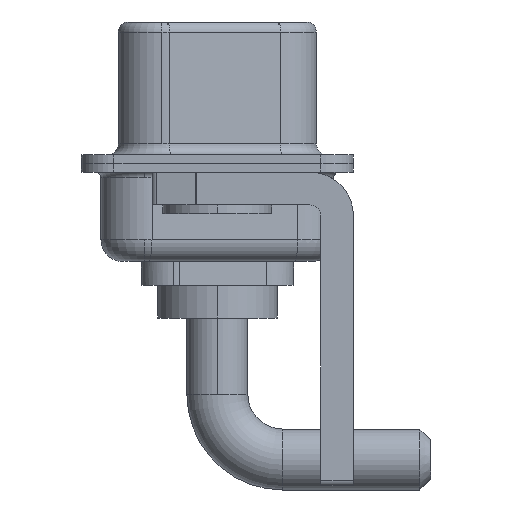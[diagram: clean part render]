
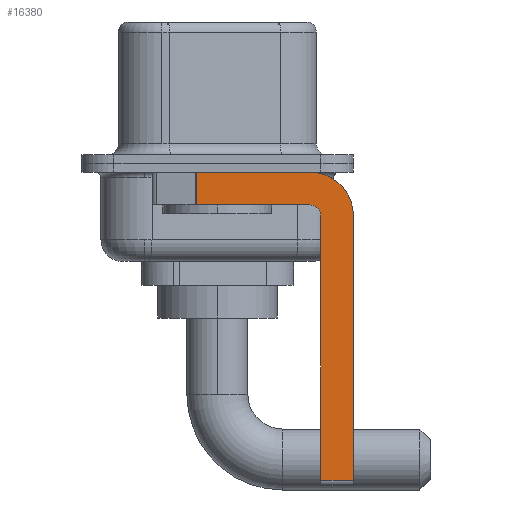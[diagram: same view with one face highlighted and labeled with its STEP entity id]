
A CAD part, left-side view. The second image highlights one B-rep face of the part: STEP entity #16380.
In plain terms, the highlighted planar face has unit normal (-1, 0, 0).
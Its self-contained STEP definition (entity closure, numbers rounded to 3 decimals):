
#33 = CARTESIAN_POINT ( 'NONE',  ( -2.9, -4.75, -14.55 ) ) ;
#86 = CIRCLE ( 'NONE', #16404, 2. ) ;
#243 = EDGE_CURVE ( 'NONE', #2593, #774, #3225, .T. ) ;
#257 = CARTESIAN_POINT ( 'NONE',  ( -2.9, -4.25, -1.9 ) ) ;
#627 = AXIS2_PLACEMENT_3D ( 'NONE', #12293, #13419, #5666 ) ;
#739 = VERTEX_POINT ( 'NONE', #6500 ) ;
#774 = VERTEX_POINT ( 'NONE', #1384 ) ;
#1222 = ORIENTED_EDGE ( 'NONE', *, *, #3602, .F. ) ;
#1384 = CARTESIAN_POINT ( 'NONE',  ( -2.9, 0.978, -1.9 ) ) ;
#1558 = ORIENTED_EDGE ( 'NONE', *, *, #5678, .F. ) ;
#1972 = VECTOR ( 'NONE', #9019, 1000. ) ;
#2199 = CARTESIAN_POINT ( 'NONE',  ( -2.9, -4.25, -2.4 ) ) ;
#2265 = VERTEX_POINT ( 'NONE', #33 ) ;
#2532 = DIRECTION ( 'NONE',  ( 0., 0., -1. ) ) ;
#2593 = VERTEX_POINT ( 'NONE', #11595 ) ;
#2694 = EDGE_CURVE ( 'NONE', #8889, #739, #14136, .T. ) ;
#3225 = LINE ( 'NONE', #7129, #10905 ) ;
#3522 = VERTEX_POINT ( 'NONE', #14858 ) ;
#3602 = EDGE_CURVE ( 'NONE', #3522, #14218, #7430, .T. ) ;
#3808 = PLANE ( 'NONE',  #4831 ) ;
#4029 = DIRECTION ( 'NONE',  ( 0., 0., -1. ) ) ;
#4514 = ORIENTED_EDGE ( 'NONE', *, *, #5252, .F. ) ;
#4831 = AXIS2_PLACEMENT_3D ( 'NONE', #2199, #8995, #2532 ) ;
#5252 = EDGE_CURVE ( 'NONE', #2593, #13153, #6380, .T. ) ;
#5563 = ORIENTED_EDGE ( 'NONE', *, *, #8252, .T. ) ;
#5666 = DIRECTION ( 'NONE',  ( 0., 0., 1. ) ) ;
#5678 = EDGE_CURVE ( 'NONE', #14218, #774, #8286, .T. ) ;
#5967 = VECTOR ( 'NONE', #7165, 1000. ) ;
#6380 = LINE ( 'NONE', #10470, #9667 ) ;
#6500 = CARTESIAN_POINT ( 'NONE',  ( -2.9, -6.25, -14.55 ) ) ;
#7129 = CARTESIAN_POINT ( 'NONE',  ( -2.9, 0.978, -1.9 ) ) ;
#7165 = DIRECTION ( 'NONE',  ( 0., 1., 0. ) ) ;
#7430 = CIRCLE ( 'NONE', #627, 0.5 ) ;
#7485 = DIRECTION ( 'NONE',  ( 0., -1., 0. ) ) ;
#8115 = ORIENTED_EDGE ( 'NONE', *, *, #243, .T. ) ;
#8252 = EDGE_CURVE ( 'NONE', #2265, #739, #16117, .T. ) ;
#8286 = LINE ( 'NONE', #16116, #5967 ) ;
#8325 = DIRECTION ( 'NONE',  ( 0., 0., 1. ) ) ;
#8410 = DIRECTION ( 'NONE',  ( 0., 0., -1. ) ) ;
#8852 = CARTESIAN_POINT ( 'NONE',  ( -2.9, -6.25, -2.4 ) ) ;
#8889 = VERTEX_POINT ( 'NONE', #10384 ) ;
#8995 = DIRECTION ( 'NONE',  ( 1., 0., 0. ) ) ;
#9019 = DIRECTION ( 'NONE',  ( 0., 0., -1. ) ) ;
#9228 = EDGE_CURVE ( 'NONE', #2265, #3522, #9599, .T. ) ;
#9484 = ORIENTED_EDGE ( 'NONE', *, *, #10272, .F. ) ;
#9599 = LINE ( 'NONE', #14800, #16662 ) ;
#9645 = CARTESIAN_POINT ( 'NONE',  ( -2.9, -4.25, -14.55 ) ) ;
#9667 = VECTOR ( 'NONE', #7485, 1000. ) ;
#10272 = EDGE_CURVE ( 'NONE', #13153, #8889, #86, .T. ) ;
#10384 = CARTESIAN_POINT ( 'NONE',  ( -2.9, -6.25, -2.4 ) ) ;
#10470 = CARTESIAN_POINT ( 'NONE',  ( -2.9, 3., -0.4 ) ) ;
#10555 = CARTESIAN_POINT ( 'NONE',  ( -2.9, -4.25, -0.4 ) ) ;
#10905 = VECTOR ( 'NONE', #8410, 1000. ) ;
#11595 = CARTESIAN_POINT ( 'NONE',  ( -2.9, 0.978, -0.4 ) ) ;
#12141 = EDGE_LOOP ( 'NONE', ( #4514, #8115, #1558, #1222, #14338, #5563, #14783, #9484 ) ) ;
#12293 = CARTESIAN_POINT ( 'NONE',  ( -2.9, -4.25, -2.4 ) ) ;
#12836 = FACE_OUTER_BOUND ( 'NONE', #12141, .T. ) ;
#13153 = VERTEX_POINT ( 'NONE', #10555 ) ;
#13419 = DIRECTION ( 'NONE',  ( -1., 0., 0. ) ) ;
#13567 = DIRECTION ( 'NONE',  ( 0., -1., 0. ) ) ;
#14077 = DIRECTION ( 'NONE',  ( 1., 0., 0. ) ) ;
#14136 = LINE ( 'NONE', #8852, #1972 ) ;
#14218 = VERTEX_POINT ( 'NONE', #257 ) ;
#14338 = ORIENTED_EDGE ( 'NONE', *, *, #9228, .F. ) ;
#14783 = ORIENTED_EDGE ( 'NONE', *, *, #2694, .F. ) ;
#14800 = CARTESIAN_POINT ( 'NONE',  ( -2.9, -4.75, -14.8 ) ) ;
#14858 = CARTESIAN_POINT ( 'NONE',  ( -2.9, -4.75, -2.4 ) ) ;
#15539 = VECTOR ( 'NONE', #13567, 1000. ) ;
#15691 = CARTESIAN_POINT ( 'NONE',  ( -2.9, -4.25, -2.4 ) ) ;
#16116 = CARTESIAN_POINT ( 'NONE',  ( -2.9, -4.25, -1.9 ) ) ;
#16117 = LINE ( 'NONE', #9645, #15539 ) ;
#16380 = ADVANCED_FACE ( 'NONE', ( #12836 ), #3808, .F. ) ;
#16404 = AXIS2_PLACEMENT_3D ( 'NONE', #15691, #14077, #4029 ) ;
#16662 = VECTOR ( 'NONE', #8325, 1000. ) ;
